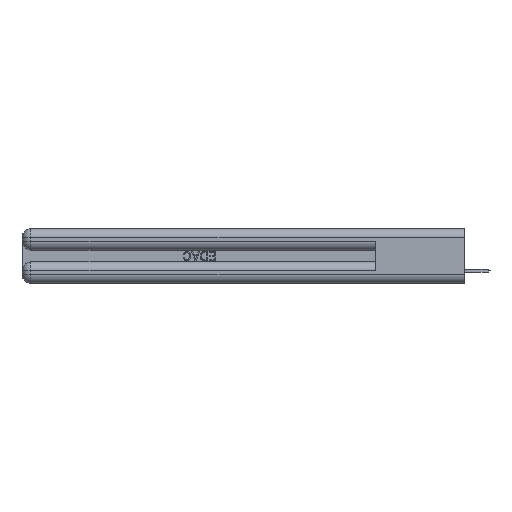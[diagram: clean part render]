
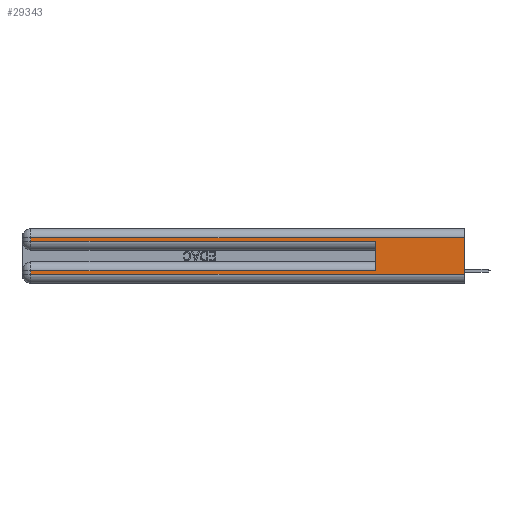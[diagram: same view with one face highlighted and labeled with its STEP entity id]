
A CAD part, left-side view. The second image highlights one B-rep face of the part: STEP entity #29343.
In plain terms, the highlighted planar face has unit normal (-1, 0, 0).
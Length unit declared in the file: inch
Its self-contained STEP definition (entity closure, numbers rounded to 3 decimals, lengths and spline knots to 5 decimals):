
#37 = LINE ( 'NONE', #13320, #26579 ) ;
#1598 = CARTESIAN_POINT ( 'NONE',  ( 0., 0., 0.31 ) ) ;
#1762 = DIRECTION ( 'NONE',  ( 0., 1., 0. ) ) ;
#2488 = VECTOR ( 'NONE', #39619, 39.37008 ) ;
#3422 = DIRECTION ( 'NONE',  ( 0., 0., -1. ) ) ;
#3559 = CARTESIAN_POINT ( 'NONE',  ( 0., 0., 0.06 ) ) ;
#3584 = PLANE ( 'NONE',  #23975 ) ;
#3783 = EDGE_CURVE ( 'NONE', #22844, #6888, #9611, .T. ) ;
#4100 = ORIENTED_EDGE ( 'NONE', *, *, #39138, .F. ) ;
#4673 = VERTEX_POINT ( 'NONE', #3559 ) ;
#5042 = EDGE_CURVE ( 'NONE', #19339, #14097, #43464, .T. ) ;
#5196 = EDGE_LOOP ( 'NONE', ( #42479, #15905, #27906, #14707, #4100, #29852, #43771, #19179 ) ) ;
#5540 = VECTOR ( 'NONE', #10742, 39.37008 ) ;
#6827 = CARTESIAN_POINT ( 'NONE',  ( 0., 0., 0.31 ) ) ;
#6888 = VERTEX_POINT ( 'NONE', #45926 ) ;
#6922 = DIRECTION ( 'NONE',  ( 0., 1., 0. ) ) ;
#7939 = VECTOR ( 'NONE', #1762, 39.37008 ) ;
#8579 = EDGE_CURVE ( 'NONE', #25990, #4673, #22833, .T. ) ;
#9137 = DIRECTION ( 'NONE',  ( 0., 0., 1. ) ) ;
#9139 = VERTEX_POINT ( 'NONE', #22119 ) ;
#9611 = LINE ( 'NONE', #21767, #26389 ) ;
#10742 = DIRECTION ( 'NONE',  ( 0., 0., -1. ) ) ;
#11885 = CARTESIAN_POINT ( 'NONE',  ( 0., 0.6, 0.085 ) ) ;
#13320 = CARTESIAN_POINT ( 'NONE',  ( 0., 0.6, 0.145 ) ) ;
#13643 = CARTESIAN_POINT ( 'NONE',  ( 0., 0., 0.37 ) ) ;
#13712 = EDGE_CURVE ( 'NONE', #14097, #32834, #39183, .T. ) ;
#14097 = VERTEX_POINT ( 'NONE', #43849 ) ;
#14291 = CARTESIAN_POINT ( 'NONE',  ( 0., 0., 0.285 ) ) ;
#14707 = ORIENTED_EDGE ( 'NONE', *, *, #13712, .T. ) ;
#15351 = EDGE_CURVE ( 'NONE', #6888, #9139, #42665, .T. ) ;
#15905 = ORIENTED_EDGE ( 'NONE', *, *, #22313, .T. ) ;
#18010 = DIRECTION ( 'NONE',  ( 0., -1., 0. ) ) ;
#18050 = DIRECTION ( 'NONE',  ( 0., 0., -1. ) ) ;
#19179 = ORIENTED_EDGE ( 'NONE', *, *, #36721, .T. ) ;
#19339 = VERTEX_POINT ( 'NONE', #47336 ) ;
#21026 = CARTESIAN_POINT ( 'NONE',  ( 0., 0., 0.06 ) ) ;
#21767 = CARTESIAN_POINT ( 'NONE',  ( 0., 0., 0.085 ) ) ;
#22119 = CARTESIAN_POINT ( 'NONE',  ( 0., 2.94, 0.06 ) ) ;
#22294 = VECTOR ( 'NONE', #18010, 39.37008 ) ;
#22313 = EDGE_CURVE ( 'NONE', #25990, #19339, #26438, .T. ) ;
#22833 = LINE ( 'NONE', #13643, #46706 ) ;
#22844 = VERTEX_POINT ( 'NONE', #11885 ) ;
#23975 = AXIS2_PLACEMENT_3D ( 'NONE', #44443, #29600, #3422 ) ;
#25990 = VERTEX_POINT ( 'NONE', #6827 ) ;
#26389 = VECTOR ( 'NONE', #6922, 39.37008 ) ;
#26438 = LINE ( 'NONE', #1598, #7939 ) ;
#26549 = VECTOR ( 'NONE', #18050, 39.37008 ) ;
#26579 = VECTOR ( 'NONE', #9137, 39.37008 ) ;
#27906 = ORIENTED_EDGE ( 'NONE', *, *, #5042, .T. ) ;
#29343 = ADVANCED_FACE ( 'NONE', ( #46206 ), #3584, .F. ) ;
#29600 = DIRECTION ( 'NONE',  ( 1., 0., 0. ) ) ;
#29852 = ORIENTED_EDGE ( 'NONE', *, *, #3783, .T. ) ;
#32678 = CARTESIAN_POINT ( 'NONE',  ( 0., 2.94, 0.37 ) ) ;
#32834 = VERTEX_POINT ( 'NONE', #42452 ) ;
#36547 = CARTESIAN_POINT ( 'NONE',  ( 0., 2.94, 0.37 ) ) ;
#36721 = EDGE_CURVE ( 'NONE', #9139, #4673, #40779, .T. ) ;
#39138 = EDGE_CURVE ( 'NONE', #22844, #32834, #37, .T. ) ;
#39183 = LINE ( 'NONE', #14291, #22294 ) ;
#39619 = DIRECTION ( 'NONE',  ( 0., -1., 0. ) ) ;
#40779 = LINE ( 'NONE', #21026, #2488 ) ;
#42452 = CARTESIAN_POINT ( 'NONE',  ( 0., 0.6, 0.285 ) ) ;
#42479 = ORIENTED_EDGE ( 'NONE', *, *, #8579, .F. ) ;
#42665 = LINE ( 'NONE', #36547, #5540 ) ;
#43058 = DIRECTION ( 'NONE',  ( 0., 0., -1. ) ) ;
#43464 = LINE ( 'NONE', #32678, #26549 ) ;
#43771 = ORIENTED_EDGE ( 'NONE', *, *, #15351, .T. ) ;
#43849 = CARTESIAN_POINT ( 'NONE',  ( 0., 2.94, 0.285 ) ) ;
#44443 = CARTESIAN_POINT ( 'NONE',  ( 0., 0., 0.37 ) ) ;
#45926 = CARTESIAN_POINT ( 'NONE',  ( 0., 2.94, 0.085 ) ) ;
#46206 = FACE_OUTER_BOUND ( 'NONE', #5196, .T. ) ;
#46706 = VECTOR ( 'NONE', #43058, 39.37008 ) ;
#47336 = CARTESIAN_POINT ( 'NONE',  ( 0., 2.94, 0.31 ) ) ;
